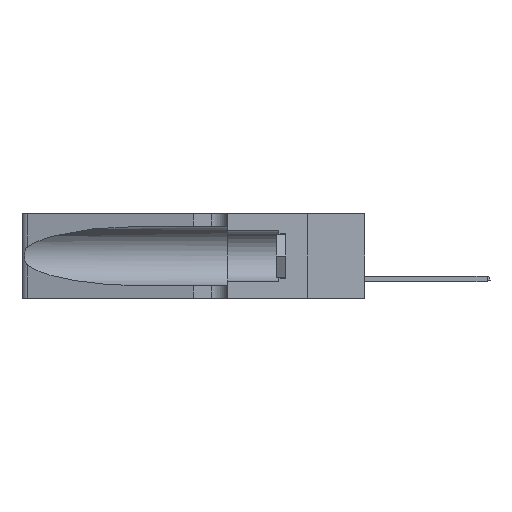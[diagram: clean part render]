
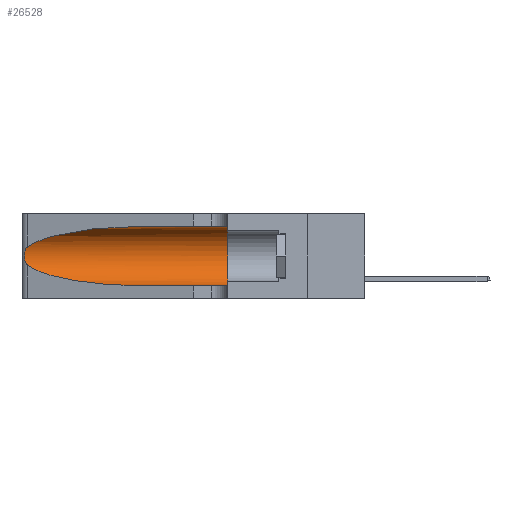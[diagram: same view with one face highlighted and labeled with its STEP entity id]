
A CAD part, left-side view. The second image highlights one B-rep face of the part: STEP entity #26528.
In plain terms, the highlighted cylindrical face has radius 3.308 mm (diameter 6.617 mm), a partial arc.
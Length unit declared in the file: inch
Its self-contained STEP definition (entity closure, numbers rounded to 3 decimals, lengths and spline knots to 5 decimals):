
#433 =( BOUNDED_CURVE ( )  B_SPLINE_CURVE ( 3, ( #19302, #24308, #11675, #1638 ),
 .UNSPECIFIED., .F., .T. ) 
 B_SPLINE_CURVE_WITH_KNOTS ( ( 4, 4 ),
 ( 1.5708, 2.84003 ),
 .UNSPECIFIED. ) 
 CURVE ( )  GEOMETRIC_REPRESENTATION_ITEM ( )  RATIONAL_B_SPLINE_CURVE ( ( 1., 0.87, 0.87, 1. ) ) 
 REPRESENTATION_ITEM ( '' )  );
#1073 = CARTESIAN_POINT ( 'NONE',  ( 0.1305, 0.35, 0.185 ) ) ;
#1555 = VERTEX_POINT ( 'NONE', #15554 ) ;
#1638 = CARTESIAN_POINT ( 'NONE',  ( 0.25487, 1.22718, 0.22369 ) ) ;
#1996 = CARTESIAN_POINT ( 'NONE',  ( 0.1305, 1.61858, 0.31525 ) ) ;
#2154 = CARTESIAN_POINT ( 'NONE',  ( 0.25555, 1.22994, 0.2215 ) ) ;
#3530 = CARTESIAN_POINT ( 'NONE',  ( 0.25487, 1.22718, 0.14631 ) ) ;
#4280 = CARTESIAN_POINT ( 'NONE',  ( 0.25639, 1.23186, 0.15144 ) ) ;
#4787 = CARTESIAN_POINT ( 'NONE',  ( 0.1305, 0.72297, 0.05475 ) ) ;
#5496 = FACE_OUTER_BOUND ( 'NONE', #5575, .T. ) ;
#5575 = EDGE_LOOP ( 'NONE', ( #26342, #21564, #7634, #19773, #30468, #24408 ) ) ;
#6312 = CARTESIAN_POINT ( 'NONE',  ( 0.1305, 0.72297, 0.31525 ) ) ;
#6703 = LINE ( 'NONE', #33096, #29975 ) ;
#6869 = CARTESIAN_POINT ( 'NONE',  ( 0.25639, 1.23184, 0.21858 ) ) ;
#7634 = ORIENTED_EDGE ( 'NONE', *, *, #27612, .T. ) ;
#8305 = DIRECTION ( 'NONE',  ( 0., -1., 0. ) ) ;
#8550 = VERTEX_POINT ( 'NONE', #4787 ) ;
#8795 = CARTESIAN_POINT ( 'NONE',  ( 0.2373, 1.15595, 0.08982 ) ) ;
#10281 = AXIS2_PLACEMENT_3D ( 'NONE', #1073, #24289, #24190 ) ;
#10314 =( BOUNDED_CURVE ( )  B_SPLINE_CURVE ( 3, ( #3530, #8795, #28869, #28980 ),
 .UNSPECIFIED., .F., .F. ) 
 B_SPLINE_CURVE_WITH_KNOTS ( ( 4, 4 ),
 ( 3.44316, 4.71239 ),
 .UNSPECIFIED. ) 
 CURVE ( )  GEOMETRIC_REPRESENTATION_ITEM ( )  RATIONAL_B_SPLINE_CURVE ( ( 1., 0.87, 0.87, 1. ) ) 
 REPRESENTATION_ITEM ( '' )  );
#10647 = LINE ( 'NONE', #1996, #25054 ) ;
#10742 = CYLINDRICAL_SURFACE ( 'NONE', #32943, 0.13025 ) ;
#11675 = CARTESIAN_POINT ( 'NONE',  ( 0.2373, 1.15595, 0.28018 ) ) ;
#12897 = VERTEX_POINT ( 'NONE', #16779 ) ;
#14516 = CARTESIAN_POINT ( 'NONE',  ( 0.26017, 1.23833, 0.17102 ) ) ;
#14856 = CARTESIAN_POINT ( 'NONE',  ( 0.26075, 1.23896, 0.178 ) ) ;
#15206 = EDGE_CURVE ( 'NONE', #23804, #16803, #21193, .T. ) ;
#15335 = EDGE_CURVE ( 'NONE', #8550, #16803, #6703, .T. ) ;
#15554 = CARTESIAN_POINT ( 'NONE',  ( 0.25487, 1.22718, 0.22369 ) ) ;
#15820 = CARTESIAN_POINT ( 'NONE',  ( 0.1305, 0.35, 0.05475 ) ) ;
#16779 = CARTESIAN_POINT ( 'NONE',  ( 0.25487, 1.22718, 0.14631 ) ) ;
#16803 = VERTEX_POINT ( 'NONE', #15820 ) ;
#17130 = CARTESIAN_POINT ( 'NONE',  ( 0.25856, 1.23593, 0.16098 ) ) ;
#17240 = CARTESIAN_POINT ( 'NONE',  ( 0.26075, 1.23896, 0.19203 ) ) ;
#17460 = CARTESIAN_POINT ( 'NONE',  ( 0.25487, 1.22718, 0.14631 ) ) ;
#18351 = B_SPLINE_CURVE_WITH_KNOTS ( 'NONE', 3,
 ( #20033, #2154, #6869, #22594, #29949, #19928, #17240, #14856, #14516, #17130, #25138, #4280, #32719, #17460 ),
 .UNSPECIFIED., .F., .F.,
 ( 4, 2, 2, 2, 2, 2, 4 ),
 ( 0., 0.00027, 0.00053, 0.00107, 0.0016, 0.00187, 0.00214 ),
 .UNSPECIFIED. ) ;
#18437 = CARTESIAN_POINT ( 'NONE',  ( 0.1305, 1.61858, 0.185 ) ) ;
#19302 = CARTESIAN_POINT ( 'NONE',  ( 0.1305, 0.72297, 0.31525 ) ) ;
#19695 = CARTESIAN_POINT ( 'NONE',  ( 0.1305, 0.35, 0.31525 ) ) ;
#19773 = ORIENTED_EDGE ( 'NONE', *, *, #15335, .T. ) ;
#19928 = CARTESIAN_POINT ( 'NONE',  ( 0.26018, 1.23835, 0.19895 ) ) ;
#20033 = CARTESIAN_POINT ( 'NONE',  ( 0.25487, 1.22718, 0.22369 ) ) ;
#20062 = EDGE_CURVE ( 'NONE', #25926, #23804, #10647, .T. ) ;
#20200 = DIRECTION ( 'NONE',  ( 0., -1., 0. ) ) ;
#21025 = DIRECTION ( 'NONE',  ( 0., 0., -1. ) ) ;
#21193 = CIRCLE ( 'NONE', #10281, 0.13025 ) ;
#21564 = ORIENTED_EDGE ( 'NONE', *, *, #27937, .T. ) ;
#22594 = CARTESIAN_POINT ( 'NONE',  ( 0.25787, 1.23484, 0.2124 ) ) ;
#23804 = VERTEX_POINT ( 'NONE', #19695 ) ;
#24190 = DIRECTION ( 'NONE',  ( 0., 0., 1. ) ) ;
#24289 = DIRECTION ( 'NONE',  ( 0., 1., 0. ) ) ;
#24308 = CARTESIAN_POINT ( 'NONE',  ( 0.18966, 0.96281, 0.31525 ) ) ;
#24408 = ORIENTED_EDGE ( 'NONE', *, *, #20062, .F. ) ;
#25054 = VECTOR ( 'NONE', #25224, 39.37008 ) ;
#25138 = CARTESIAN_POINT ( 'NONE',  ( 0.25789, 1.23486, 0.15765 ) ) ;
#25224 = DIRECTION ( 'NONE',  ( 0., -1., 0. ) ) ;
#25926 = VERTEX_POINT ( 'NONE', #6312 ) ;
#26342 = ORIENTED_EDGE ( 'NONE', *, *, #31758, .T. ) ;
#26528 = ADVANCED_FACE ( 'NONE', ( #5496 ), #10742, .F. ) ;
#27612 = EDGE_CURVE ( 'NONE', #12897, #8550, #10314, .T. ) ;
#27937 = EDGE_CURVE ( 'NONE', #1555, #12897, #18351, .T. ) ;
#28869 = CARTESIAN_POINT ( 'NONE',  ( 0.18966, 0.96281, 0.05475 ) ) ;
#28980 = CARTESIAN_POINT ( 'NONE',  ( 0.1305, 0.72297, 0.05475 ) ) ;
#29949 = CARTESIAN_POINT ( 'NONE',  ( 0.25854, 1.2359, 0.20912 ) ) ;
#29975 = VECTOR ( 'NONE', #20200, 39.37008 ) ;
#30468 = ORIENTED_EDGE ( 'NONE', *, *, #15206, .F. ) ;
#31758 = EDGE_CURVE ( 'NONE', #25926, #1555, #433, .T. ) ;
#32719 = CARTESIAN_POINT ( 'NONE',  ( 0.25555, 1.22993, 0.14849 ) ) ;
#32943 = AXIS2_PLACEMENT_3D ( 'NONE', #18437, #8305, #21025 ) ;
#33096 = CARTESIAN_POINT ( 'NONE',  ( 0.1305, 1.61858, 0.05475 ) ) ;
